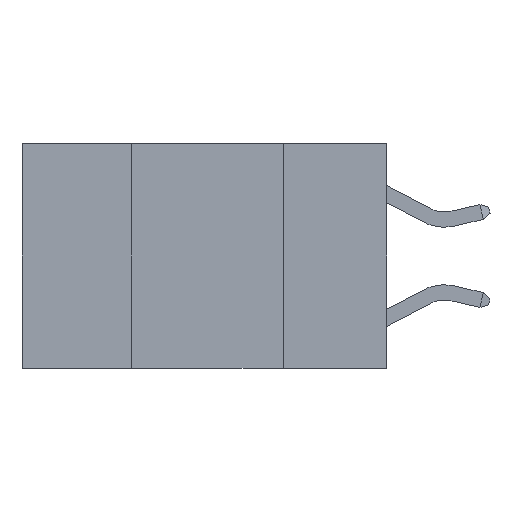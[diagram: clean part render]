
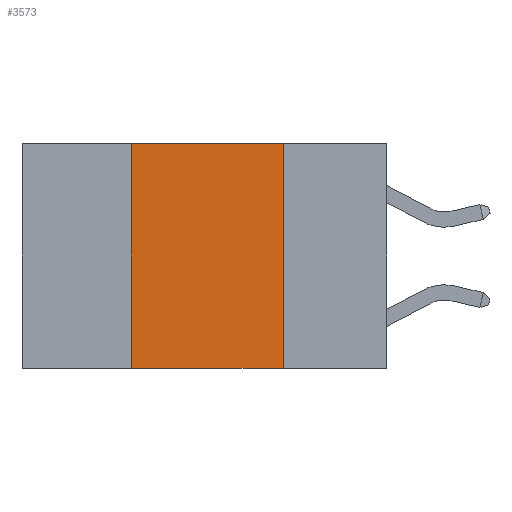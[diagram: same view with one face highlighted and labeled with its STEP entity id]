
A CAD part, left-side view. The second image highlights one B-rep face of the part: STEP entity #3573.
In plain terms, the highlighted planar face has unit normal (-1, 0, 0).
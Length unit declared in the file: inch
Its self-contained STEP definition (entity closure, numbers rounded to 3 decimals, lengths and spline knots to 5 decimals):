
#15 = DIRECTION ( 'NONE',  ( 1., 0., 0. ) ) ;
#644 = DIRECTION ( 'NONE',  ( 0., 0., -1. ) ) ;
#1218 = EDGE_CURVE ( 'NONE', #7969, #5619, #4023, .T. ) ;
#1336 = ORIENTED_EDGE ( 'NONE', *, *, #2312, .F. ) ;
#1513 = LINE ( 'NONE', #5715, #1935 ) ;
#1546 = VERTEX_POINT ( 'NONE', #5792 ) ;
#1935 = VECTOR ( 'NONE', #7166, 39.37008 ) ;
#1955 = CARTESIAN_POINT ( 'NONE',  ( 0., 0.42, 0. ) ) ;
#2312 = EDGE_CURVE ( 'NONE', #1546, #2816, #6954, .T. ) ;
#2347 = DIRECTION ( 'NONE',  ( 0., -1., 0. ) ) ;
#2816 = VERTEX_POINT ( 'NONE', #4892 ) ;
#3058 = EDGE_CURVE ( 'NONE', #7969, #2816, #4653, .T. ) ;
#3072 = VECTOR ( 'NONE', #644, 39.37008 ) ;
#3090 = VECTOR ( 'NONE', #5002, 39.37008 ) ;
#3519 = DIRECTION ( 'NONE',  ( 0., 0., -1. ) ) ;
#3573 = ADVANCED_FACE ( 'NONE', ( #8996 ), #5317, .F. ) ;
#3689 = VECTOR ( 'NONE', #2347, 39.37008 ) ;
#3872 = CARTESIAN_POINT ( 'NONE',  ( 0., 0.42, 0. ) ) ;
#3896 = CARTESIAN_POINT ( 'NONE',  ( 0., 0.42, -0.37 ) ) ;
#4023 = LINE ( 'NONE', #1955, #3090 ) ;
#4132 = EDGE_CURVE ( 'NONE', #5619, #1546, #1513, .T. ) ;
#4477 = ORIENTED_EDGE ( 'NONE', *, *, #1218, .F. ) ;
#4637 = ORIENTED_EDGE ( 'NONE', *, *, #3058, .T. ) ;
#4653 = LINE ( 'NONE', #7298, #3689 ) ;
#4892 = CARTESIAN_POINT ( 'NONE',  ( 0., 0.17, -0.37 ) ) ;
#5002 = DIRECTION ( 'NONE',  ( 0., 0., 1. ) ) ;
#5162 = AXIS2_PLACEMENT_3D ( 'NONE', #8814, #15, #3519 ) ;
#5317 = PLANE ( 'NONE',  #5162 ) ;
#5619 = VERTEX_POINT ( 'NONE', #3872 ) ;
#5715 = CARTESIAN_POINT ( 'NONE',  ( 0., 0.6, 0. ) ) ;
#5792 = CARTESIAN_POINT ( 'NONE',  ( 0., 0.17, 0. ) ) ;
#6362 = CARTESIAN_POINT ( 'NONE',  ( 0., 0.17, 0. ) ) ;
#6954 = LINE ( 'NONE', #6362, #3072 ) ;
#7166 = DIRECTION ( 'NONE',  ( 0., -1., 0. ) ) ;
#7298 = CARTESIAN_POINT ( 'NONE',  ( 0., 0.6, -0.37 ) ) ;
#7678 = ORIENTED_EDGE ( 'NONE', *, *, #4132, .F. ) ;
#7969 = VERTEX_POINT ( 'NONE', #3896 ) ;
#8814 = CARTESIAN_POINT ( 'NONE',  ( 0., 0.6, 0. ) ) ;
#8996 = FACE_OUTER_BOUND ( 'NONE', #9056, .T. ) ;
#9056 = EDGE_LOOP ( 'NONE', ( #1336, #7678, #4477, #4637 ) ) ;
